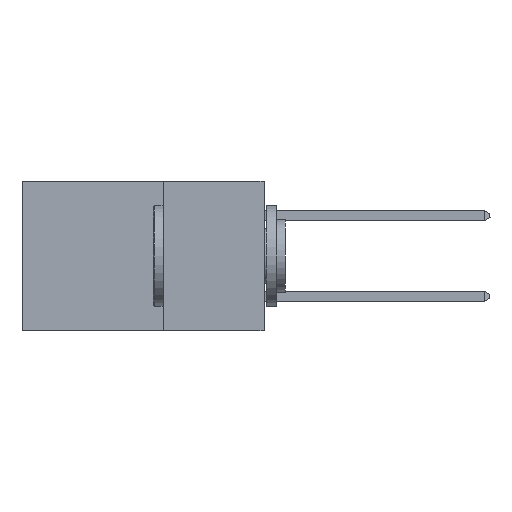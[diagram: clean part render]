
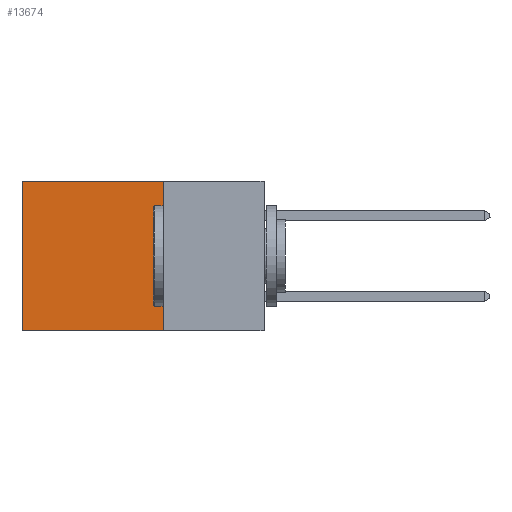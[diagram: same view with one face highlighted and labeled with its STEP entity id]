
A CAD part, left-side view. The second image highlights one B-rep face of the part: STEP entity #13674.
In plain terms, the highlighted planar face has unit normal (-1, 0, 0).
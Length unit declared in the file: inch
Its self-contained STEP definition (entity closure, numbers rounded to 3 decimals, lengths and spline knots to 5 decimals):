
#13 = AXIS2_PLACEMENT_3D ( 'NONE', #9518, #9465, #286 ) ;
#213 = ORIENTED_EDGE ( 'NONE', *, *, #1717, .F. ) ;
#286 = DIRECTION ( 'NONE',  ( 0., 0., -1. ) ) ;
#1589 = VECTOR ( 'NONE', #3702, 39.37008 ) ;
#1690 = CARTESIAN_POINT ( 'NONE',  ( 0.298, 0.25, 0. ) ) ;
#1717 = EDGE_CURVE ( 'NONE', #8141, #12575, #13582, .T. ) ;
#2314 = LINE ( 'NONE', #9424, #1589 ) ;
#2568 = EDGE_CURVE ( 'NONE', #12814, #8141, #2314, .T. ) ;
#3116 = VERTEX_POINT ( 'NONE', #13291 ) ;
#3702 = DIRECTION ( 'NONE',  ( 0., 0., -1. ) ) ;
#4711 = DIRECTION ( 'NONE',  ( 0., 1., 0. ) ) ;
#4764 = EDGE_CURVE ( 'NONE', #12814, #3116, #11421, .T. ) ;
#5010 = CARTESIAN_POINT ( 'NONE',  ( 0.298, 0.6, -0.37 ) ) ;
#6133 = PLANE ( 'NONE',  #13 ) ;
#6740 = CARTESIAN_POINT ( 'NONE',  ( 0.298, 0.6, 0. ) ) ;
#7013 = VECTOR ( 'NONE', #8973, 39.37008 ) ;
#7563 = LINE ( 'NONE', #6740, #7013 ) ;
#8141 = VERTEX_POINT ( 'NONE', #14087 ) ;
#8177 = ORIENTED_EDGE ( 'NONE', *, *, #2568, .F. ) ;
#8973 = DIRECTION ( 'NONE',  ( 0., 0., -1. ) ) ;
#8974 = VECTOR ( 'NONE', #10306, 39.37008 ) ;
#9187 = CARTESIAN_POINT ( 'NONE',  ( 0.298, 0.25, 0. ) ) ;
#9424 = CARTESIAN_POINT ( 'NONE',  ( 0.298, 0.25, 0. ) ) ;
#9465 = DIRECTION ( 'NONE',  ( 1., 0., 0. ) ) ;
#9518 = CARTESIAN_POINT ( 'NONE',  ( 0.298, 0.25, 0. ) ) ;
#10306 = DIRECTION ( 'NONE',  ( 0., 1., 0. ) ) ;
#10660 = EDGE_CURVE ( 'NONE', #3116, #12575, #7563, .T. ) ;
#11303 = CARTESIAN_POINT ( 'NONE',  ( 0.298, 0.25, -0.37 ) ) ;
#11421 = LINE ( 'NONE', #9187, #8974 ) ;
#11889 = ORIENTED_EDGE ( 'NONE', *, *, #10660, .T. ) ;
#11932 = VECTOR ( 'NONE', #4711, 39.37008 ) ;
#12575 = VERTEX_POINT ( 'NONE', #5010 ) ;
#12666 = EDGE_LOOP ( 'NONE', ( #11889, #213, #8177, #14334 ) ) ;
#12814 = VERTEX_POINT ( 'NONE', #1690 ) ;
#13291 = CARTESIAN_POINT ( 'NONE',  ( 0.298, 0.6, 0. ) ) ;
#13582 = LINE ( 'NONE', #11303, #11932 ) ;
#13674 = ADVANCED_FACE ( 'NONE', ( #14952 ), #6133, .F. ) ;
#14087 = CARTESIAN_POINT ( 'NONE',  ( 0.298, 0.25, -0.37 ) ) ;
#14334 = ORIENTED_EDGE ( 'NONE', *, *, #4764, .T. ) ;
#14952 = FACE_OUTER_BOUND ( 'NONE', #12666, .T. ) ;
